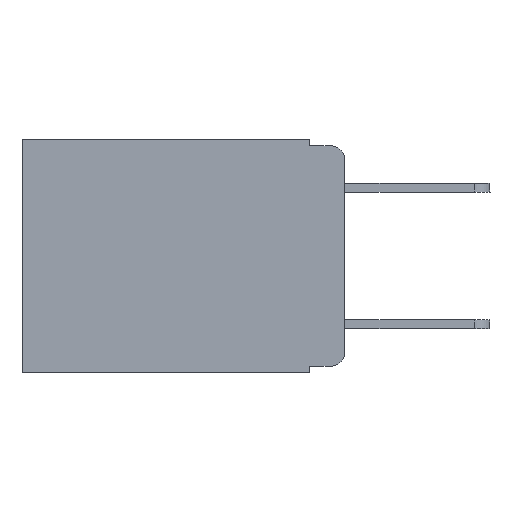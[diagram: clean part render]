
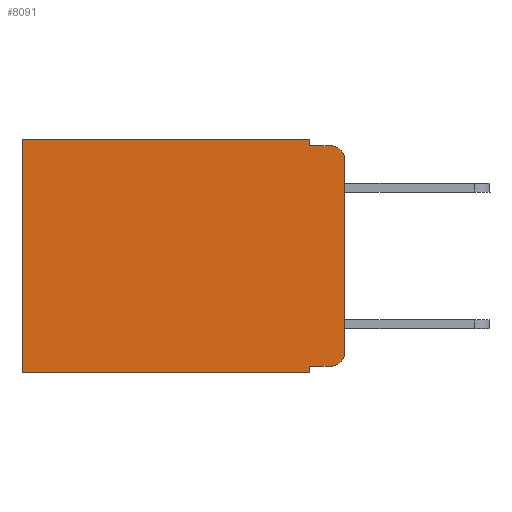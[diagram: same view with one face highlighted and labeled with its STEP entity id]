
A CAD part, left-side view. The second image highlights one B-rep face of the part: STEP entity #8091.
In plain terms, the highlighted planar face has unit normal (-1, 0, 0).
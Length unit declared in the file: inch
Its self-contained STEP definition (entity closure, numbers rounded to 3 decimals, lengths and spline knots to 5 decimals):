
#225 = EDGE_CURVE ( 'NONE', #2535, #16504, #7183, .T. ) ;
#821 = VECTOR ( 'NONE', #13863, 39.37008 ) ;
#864 = EDGE_CURVE ( 'NONE', #11175, #2535, #10527, .T. ) ;
#1320 = ORIENTED_EDGE ( 'NONE', *, *, #225, .F. ) ;
#1471 = ORIENTED_EDGE ( 'NONE', *, *, #5299, .T. ) ;
#1502 = EDGE_CURVE ( 'NONE', #1890, #16504, #5094, .T. ) ;
#1656 = CARTESIAN_POINT ( 'NONE',  ( 0.298, 0., -0.03 ) ) ;
#1890 = VERTEX_POINT ( 'NONE', #1656 ) ;
#1956 = VECTOR ( 'NONE', #13858, 39.37008 ) ;
#2325 = CARTESIAN_POINT ( 'NONE',  ( 0.298, 0.473, 0. ) ) ;
#2535 = VERTEX_POINT ( 'NONE', #14172 ) ;
#2828 = VERTEX_POINT ( 'NONE', #11189 ) ;
#3102 = AXIS2_PLACEMENT_3D ( 'NONE', #4035, #16949, #13030 ) ;
#3222 = CARTESIAN_POINT ( 'NONE',  ( 0.298, 0.02, -0.333 ) ) ;
#3274 = DIRECTION ( 'NONE',  ( 0., 1., 0. ) ) ;
#3283 = LINE ( 'NONE', #8556, #1956 ) ;
#3694 = VECTOR ( 'NONE', #3274, 39.37008 ) ;
#3815 = CARTESIAN_POINT ( 'NONE',  ( 0.298, 0., -0.313 ) ) ;
#4035 = CARTESIAN_POINT ( 'NONE',  ( 0.298, 0.02, -0.313 ) ) ;
#4107 = EDGE_CURVE ( 'NONE', #1890, #15668, #5712, .T. ) ;
#4139 = CARTESIAN_POINT ( 'NONE',  ( 0.298, 0.051, -0.343 ) ) ;
#4254 = AXIS2_PLACEMENT_3D ( 'NONE', #16575, #9977, #15262 ) ;
#4257 = DIRECTION ( 'NONE',  ( -1., 0., 0. ) ) ;
#4402 = CARTESIAN_POINT ( 'NONE',  ( 0.298, 0., -0.343 ) ) ;
#4411 = EDGE_LOOP ( 'NONE', ( #4569, #8562, #1320, #10696, #7961, #1471, #5168, #12592, #12689, #14552 ) ) ;
#4521 = CARTESIAN_POINT ( 'NONE',  ( 0.298, 0.02, -0.03 ) ) ;
#4569 = ORIENTED_EDGE ( 'NONE', *, *, #4107, .F. ) ;
#5094 = CIRCLE ( 'NONE', #7858, 0.02 ) ;
#5158 = EDGE_CURVE ( 'NONE', #16216, #14869, #9026, .T. ) ;
#5168 = ORIENTED_EDGE ( 'NONE', *, *, #16859, .F. ) ;
#5221 = VERTEX_POINT ( 'NONE', #3222 ) ;
#5253 = CARTESIAN_POINT ( 'NONE',  ( 0.298, 0.051, 0. ) ) ;
#5299 = EDGE_CURVE ( 'NONE', #6058, #2828, #9270, .T. ) ;
#5568 = CIRCLE ( 'NONE', #3102, 0.02 ) ;
#5712 = LINE ( 'NONE', #15087, #821 ) ;
#6058 = VERTEX_POINT ( 'NONE', #2325 ) ;
#6921 = DIRECTION ( 'NONE',  ( 0., 0., -1. ) ) ;
#7183 = LINE ( 'NONE', #15099, #12850 ) ;
#7792 = CARTESIAN_POINT ( 'NONE',  ( 0.298, 0.051, 0. ) ) ;
#7858 = AXIS2_PLACEMENT_3D ( 'NONE', #4521, #4257, #6921 ) ;
#7961 = ORIENTED_EDGE ( 'NONE', *, *, #12146, .T. ) ;
#8091 = ADVANCED_FACE ( 'NONE', ( #15432 ), #11097, .F. ) ;
#8287 = LINE ( 'NONE', #4402, #3694 ) ;
#8556 = CARTESIAN_POINT ( 'NONE',  ( 0.298, 0.051, -0.333 ) ) ;
#8562 = ORIENTED_EDGE ( 'NONE', *, *, #1502, .T. ) ;
#9026 = LINE ( 'NONE', #7792, #13009 ) ;
#9270 = LINE ( 'NONE', #13507, #11092 ) ;
#9542 = LINE ( 'NONE', #14840, #13864 ) ;
#9888 = EDGE_CURVE ( 'NONE', #16216, #5221, #3283, .T. ) ;
#9977 = DIRECTION ( 'NONE',  ( 1., 0., 0. ) ) ;
#10527 = LINE ( 'NONE', #17024, #16147 ) ;
#10696 = ORIENTED_EDGE ( 'NONE', *, *, #864, .F. ) ;
#11092 = VECTOR ( 'NONE', #11784, 39.37008 ) ;
#11097 = PLANE ( 'NONE',  #4254 ) ;
#11175 = VERTEX_POINT ( 'NONE', #5253 ) ;
#11189 = CARTESIAN_POINT ( 'NONE',  ( 0.298, 0.473, -0.343 ) ) ;
#11784 = DIRECTION ( 'NONE',  ( 0., 0., -1. ) ) ;
#12146 = EDGE_CURVE ( 'NONE', #11175, #6058, #9542, .T. ) ;
#12592 = ORIENTED_EDGE ( 'NONE', *, *, #5158, .F. ) ;
#12689 = ORIENTED_EDGE ( 'NONE', *, *, #9888, .T. ) ;
#12850 = VECTOR ( 'NONE', #14047, 39.37008 ) ;
#13009 = VECTOR ( 'NONE', #15521, 39.37008 ) ;
#13030 = DIRECTION ( 'NONE',  ( 0., 0., -1. ) ) ;
#13407 = EDGE_CURVE ( 'NONE', #5221, #15668, #5568, .T. ) ;
#13507 = CARTESIAN_POINT ( 'NONE',  ( 0.298, 0.473, 0. ) ) ;
#13508 = CARTESIAN_POINT ( 'NONE',  ( 0.298, 0.02, -0.01 ) ) ;
#13858 = DIRECTION ( 'NONE',  ( 0., -1., 0. ) ) ;
#13863 = DIRECTION ( 'NONE',  ( 0., 0., -1. ) ) ;
#13864 = VECTOR ( 'NONE', #15006, 39.37008 ) ;
#14047 = DIRECTION ( 'NONE',  ( 0., -1., 0. ) ) ;
#14172 = CARTESIAN_POINT ( 'NONE',  ( 0.298, 0.051, -0.01 ) ) ;
#14419 = DIRECTION ( 'NONE',  ( 0., 0., -1. ) ) ;
#14552 = ORIENTED_EDGE ( 'NONE', *, *, #13407, .T. ) ;
#14840 = CARTESIAN_POINT ( 'NONE',  ( 0.298, 0., 0. ) ) ;
#14869 = VERTEX_POINT ( 'NONE', #4139 ) ;
#14977 = CARTESIAN_POINT ( 'NONE',  ( 0.298, 0.051, -0.333 ) ) ;
#15006 = DIRECTION ( 'NONE',  ( 0., 1., 0. ) ) ;
#15087 = CARTESIAN_POINT ( 'NONE',  ( 0.298, 0., 0. ) ) ;
#15099 = CARTESIAN_POINT ( 'NONE',  ( 0.298, 0.051, -0.01 ) ) ;
#15262 = DIRECTION ( 'NONE',  ( 0., 0., -1. ) ) ;
#15432 = FACE_OUTER_BOUND ( 'NONE', #4411, .T. ) ;
#15521 = DIRECTION ( 'NONE',  ( 0., 0., -1. ) ) ;
#15668 = VERTEX_POINT ( 'NONE', #3815 ) ;
#16147 = VECTOR ( 'NONE', #14419, 39.37008 ) ;
#16216 = VERTEX_POINT ( 'NONE', #14977 ) ;
#16504 = VERTEX_POINT ( 'NONE', #13508 ) ;
#16575 = CARTESIAN_POINT ( 'NONE',  ( 0.298, 0., 0. ) ) ;
#16859 = EDGE_CURVE ( 'NONE', #14869, #2828, #8287, .T. ) ;
#16949 = DIRECTION ( 'NONE',  ( -1., 0., 0. ) ) ;
#17024 = CARTESIAN_POINT ( 'NONE',  ( 0.298, 0.051, 0. ) ) ;
